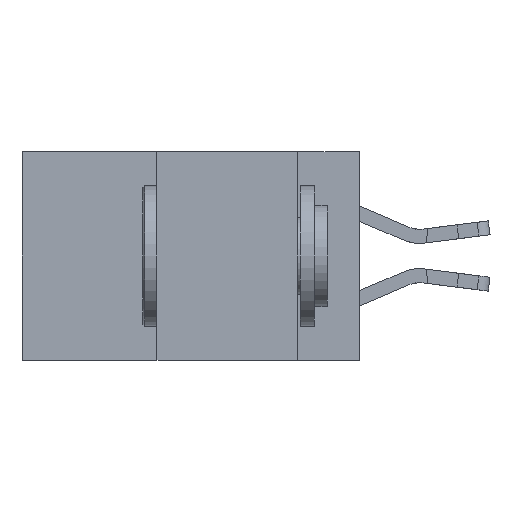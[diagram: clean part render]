
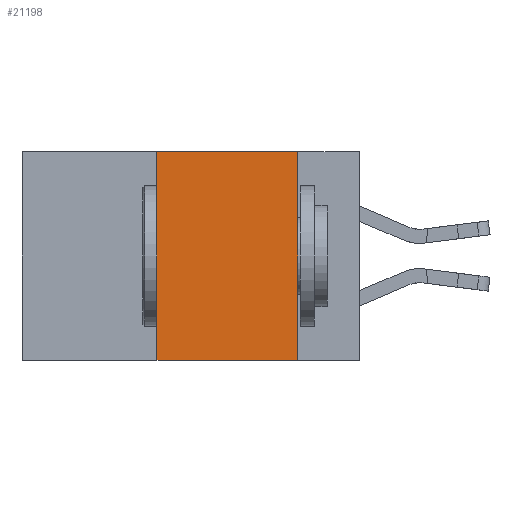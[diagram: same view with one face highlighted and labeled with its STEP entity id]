
A CAD part, left-side view. The second image highlights one B-rep face of the part: STEP entity #21198.
In plain terms, the highlighted planar face has unit normal (-1, 0, 0).
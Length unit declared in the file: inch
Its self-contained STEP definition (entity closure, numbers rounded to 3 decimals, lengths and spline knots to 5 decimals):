
#650 = DIRECTION ( 'NONE',  ( 0., -1., 0. ) ) ;
#1360 = VERTEX_POINT ( 'NONE', #2070 ) ;
#2070 = CARTESIAN_POINT ( 'NONE',  ( 0., 0.11, -0.37 ) ) ;
#2170 = CARTESIAN_POINT ( 'NONE',  ( 0., 0.36, 0. ) ) ;
#2205 = DIRECTION ( 'NONE',  ( 0., 0., 1. ) ) ;
#3557 = EDGE_CURVE ( 'NONE', #5510, #27569, #24244, .T. ) ;
#4303 = LINE ( 'NONE', #8473, #20597 ) ;
#4572 = LINE ( 'NONE', #18419, #26514 ) ;
#5510 = VERTEX_POINT ( 'NONE', #5636 ) ;
#5636 = CARTESIAN_POINT ( 'NONE',  ( 0., 0.36, -0.37 ) ) ;
#5813 = EDGE_CURVE ( 'NONE', #27569, #7542, #4572, .T. ) ;
#6593 = AXIS2_PLACEMENT_3D ( 'NONE', #14639, #12580, #27387 ) ;
#6777 = EDGE_LOOP ( 'NONE', ( #20100, #10155, #15788, #22097 ) ) ;
#7068 = CARTESIAN_POINT ( 'NONE',  ( 0., 0.6, -0.37 ) ) ;
#7542 = VERTEX_POINT ( 'NONE', #20785 ) ;
#7560 = CARTESIAN_POINT ( 'NONE',  ( 0., 0.36, 0. ) ) ;
#8473 = CARTESIAN_POINT ( 'NONE',  ( 0., 0.11, 0. ) ) ;
#10155 = ORIENTED_EDGE ( 'NONE', *, *, #5813, .F. ) ;
#10935 = VECTOR ( 'NONE', #650, 39.37008 ) ;
#12264 = LINE ( 'NONE', #7068, #10935 ) ;
#12580 = DIRECTION ( 'NONE',  ( 1., 0., 0. ) ) ;
#12968 = VECTOR ( 'NONE', #2205, 39.37008 ) ;
#14639 = CARTESIAN_POINT ( 'NONE',  ( 0., 0.6, 0. ) ) ;
#14875 = DIRECTION ( 'NONE',  ( 0., 0., -1. ) ) ;
#15788 = ORIENTED_EDGE ( 'NONE', *, *, #3557, .F. ) ;
#15959 = EDGE_CURVE ( 'NONE', #5510, #1360, #12264, .T. ) ;
#18419 = CARTESIAN_POINT ( 'NONE',  ( 0., 0.6, 0. ) ) ;
#20100 = ORIENTED_EDGE ( 'NONE', *, *, #26559, .F. ) ;
#20597 = VECTOR ( 'NONE', #14875, 39.37008 ) ;
#20785 = CARTESIAN_POINT ( 'NONE',  ( 0., 0.11, 0. ) ) ;
#21198 = ADVANCED_FACE ( 'NONE', ( #23759 ), #25275, .F. ) ;
#22097 = ORIENTED_EDGE ( 'NONE', *, *, #15959, .T. ) ;
#22683 = DIRECTION ( 'NONE',  ( 0., -1., 0. ) ) ;
#23759 = FACE_OUTER_BOUND ( 'NONE', #6777, .T. ) ;
#24244 = LINE ( 'NONE', #2170, #12968 ) ;
#25275 = PLANE ( 'NONE',  #6593 ) ;
#26514 = VECTOR ( 'NONE', #22683, 39.37008 ) ;
#26559 = EDGE_CURVE ( 'NONE', #7542, #1360, #4303, .T. ) ;
#27387 = DIRECTION ( 'NONE',  ( 0., 0., -1. ) ) ;
#27569 = VERTEX_POINT ( 'NONE', #7560 ) ;
